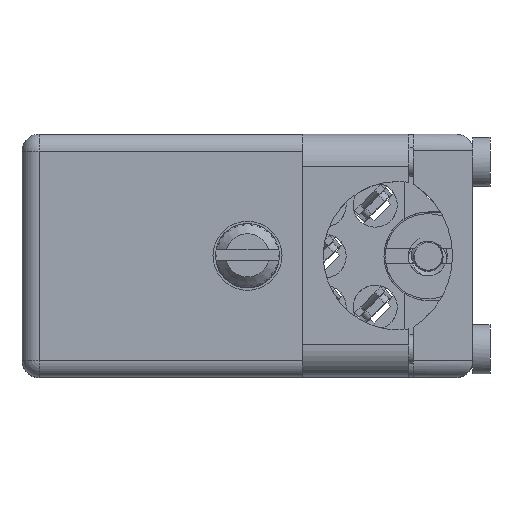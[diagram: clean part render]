
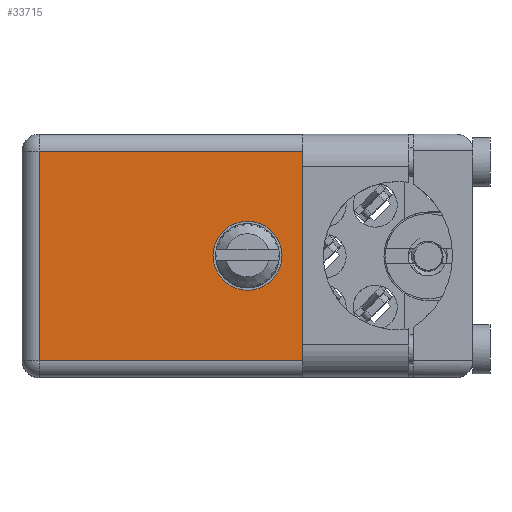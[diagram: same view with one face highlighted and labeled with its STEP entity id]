
A CAD part, top view. The second image highlights one B-rep face of the part: STEP entity #33715.
In plain terms, the highlighted face is planar.
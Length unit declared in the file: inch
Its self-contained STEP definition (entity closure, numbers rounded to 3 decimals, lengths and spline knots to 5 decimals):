
#2280 = VECTOR ( 'NONE', #78343, 39.37008 ) ;
#4469 = AXIS2_PLACEMENT_3D ( 'NONE', #117128, #179410, #145827 ) ;
#11707 = VECTOR ( 'NONE', #194479, 39.37008 ) ;
#15345 = ORIENTED_EDGE ( 'NONE', *, *, #191166, .F. ) ;
#16782 = ORIENTED_EDGE ( 'NONE', *, *, #192818, .F. ) ;
#17512 = AXIS2_PLACEMENT_3D ( 'NONE', #48209, #168682, #169655 ) ;
#18104 = CARTESIAN_POINT ( 'NONE',  ( 0., 0.906, -0.665 ) ) ;
#18209 = CARTESIAN_POINT ( 'NONE',  ( 0.05, 0.906, -0.715 ) ) ;
#19798 = CIRCLE ( 'NONE', #4469, 0.1015 ) ;
#19978 = VECTOR ( 'NONE', #87332, 39.37008 ) ;
#22488 = VERTEX_POINT ( 'NONE', #194819 ) ;
#24714 = LINE ( 'NONE', #98712, #146608 ) ;
#26294 = VERTEX_POINT ( 'NONE', #91456 ) ;
#27596 = LINE ( 'NONE', #102563, #11707 ) ;
#33715 = ADVANCED_FACE ( 'NONE', ( #63022, #94491 ), #183495, .T. ) ;
#39532 = DIRECTION ( 'NONE',  ( 0., 0., 1. ) ) ;
#39590 = CIRCLE ( 'NONE', #86900, 0.1015 ) ;
#40896 = VERTEX_POINT ( 'NONE', #136985 ) ;
#42227 = CARTESIAN_POINT ( 'NONE',  ( 0.05, 0.906, -0.05 ) ) ;
#43922 = LINE ( 'NONE', #132750, #19978 ) ;
#44995 = ORIENTED_EDGE ( 'NONE', *, *, #147206, .T. ) ;
#45551 = ORIENTED_EDGE ( 'NONE', *, *, #162852, .T. ) ;
#46807 = VECTOR ( 'NONE', #107483, 39.37008 ) ;
#46861 = LINE ( 'NONE', #169249, #115347 ) ;
#48209 = CARTESIAN_POINT ( 'NONE',  ( 0., 0.906, -0.715 ) ) ;
#51834 = DIRECTION ( 'NONE',  ( 1., 0., 0. ) ) ;
#62132 = LINE ( 'NONE', #122316, #46807 ) ;
#62166 = CARTESIAN_POINT ( 'NONE',  ( 1.15, 0.906, -0.6025 ) ) ;
#63022 = FACE_OUTER_BOUND ( 'NONE', #148347, .T. ) ;
#70532 = CARTESIAN_POINT ( 'NONE',  ( 1.15, 0.906, -0.05 ) ) ;
#73700 = VECTOR ( 'NONE', #51834, 39.37008 ) ;
#76303 = DIRECTION ( 'NONE',  ( 0., 0., 1. ) ) ;
#76359 = EDGE_CURVE ( 'NONE', #112661, #138164, #27596, .T. ) ;
#78343 = DIRECTION ( 'NONE',  ( -1., 0., 0. ) ) ;
#79406 = VERTEX_POINT ( 'NONE', #148824 ) ;
#80008 = VECTOR ( 'NONE', #141597, 39.37008 ) ;
#80374 = LINE ( 'NONE', #18209, #80008 ) ;
#84401 = CARTESIAN_POINT ( 'NONE',  ( 1.15, 0.906, -0.1125 ) ) ;
#84793 = ORIENTED_EDGE ( 'NONE', *, *, #152668, .F. ) ;
#85545 = VERTEX_POINT ( 'NONE', #157848 ) ;
#86900 = AXIS2_PLACEMENT_3D ( 'NONE', #109773, #125562, #76303 ) ;
#87332 = DIRECTION ( 'NONE',  ( 1., 0., 0. ) ) ;
#91456 = CARTESIAN_POINT ( 'NONE',  ( 0.865, 0.906, -0.6025 ) ) ;
#93102 = LINE ( 'NONE', #18104, #2280 ) ;
#93901 = ORIENTED_EDGE ( 'NONE', *, *, #76359, .T. ) ;
#94491 = FACE_BOUND ( 'NONE', #98132, .T. ) ;
#98132 = EDGE_LOOP ( 'NONE', ( #165272, #15345 ) ) ;
#98712 = CARTESIAN_POINT ( 'NONE',  ( 1.15, 0.906, -0.715 ) ) ;
#102563 = CARTESIAN_POINT ( 'NONE',  ( 0.865, 0.906, -0.1125 ) ) ;
#105263 = ORIENTED_EDGE ( 'NONE', *, *, #132419, .T. ) ;
#107483 = DIRECTION ( 'NONE',  ( 0., 0., -1. ) ) ;
#109773 = CARTESIAN_POINT ( 'NONE',  ( 0.6625, 0.906, -0.3575 ) ) ;
#112661 = VERTEX_POINT ( 'NONE', #84401 ) ;
#115347 = VECTOR ( 'NONE', #184052, 39.37008 ) ;
#117128 = CARTESIAN_POINT ( 'NONE',  ( 0.6625, 0.906, -0.3575 ) ) ;
#118645 = EDGE_CURVE ( 'NONE', #138164, #26294, #62132, .T. ) ;
#122316 = CARTESIAN_POINT ( 'NONE',  ( 0.865, 0.906, -0.1125 ) ) ;
#125562 = DIRECTION ( 'NONE',  ( 0., 1., 0. ) ) ;
#129329 = EDGE_CURVE ( 'NONE', #182599, #40896, #160449, .T. ) ;
#132419 = EDGE_CURVE ( 'NONE', #143278, #182599, #80374, .T. ) ;
#132750 = CARTESIAN_POINT ( 'NONE',  ( 0.865, 0.906, -0.6025 ) ) ;
#136495 = ORIENTED_EDGE ( 'NONE', *, *, #118645, .T. ) ;
#136985 = CARTESIAN_POINT ( 'NONE',  ( 1.15, 0.906, -0.05 ) ) ;
#138164 = VERTEX_POINT ( 'NONE', #168419 ) ;
#141597 = DIRECTION ( 'NONE',  ( 0., 0., 1. ) ) ;
#143278 = VERTEX_POINT ( 'NONE', #155475 ) ;
#145827 = DIRECTION ( 'NONE',  ( 0., 0., 1. ) ) ;
#146608 = VECTOR ( 'NONE', #39532, 39.37008 ) ;
#147206 = EDGE_CURVE ( 'NONE', #26294, #183003, #43922, .T. ) ;
#148347 = EDGE_LOOP ( 'NONE', ( #105263, #151082, #16782, #93901, #136495, #44995, #84793, #45551 ) ) ;
#148824 = CARTESIAN_POINT ( 'NONE',  ( 0.6625, 0.906, -0.459 ) ) ;
#151082 = ORIENTED_EDGE ( 'NONE', *, *, #129329, .T. ) ;
#152668 = EDGE_CURVE ( 'NONE', #22488, #183003, #24714, .T. ) ;
#155475 = CARTESIAN_POINT ( 'NONE',  ( 0.05, 0.906, -0.665 ) ) ;
#157848 = CARTESIAN_POINT ( 'NONE',  ( 0.6625, 0.906, -0.256 ) ) ;
#160449 = LINE ( 'NONE', #70532, #73700 ) ;
#162852 = EDGE_CURVE ( 'NONE', #22488, #143278, #93102, .T. ) ;
#165272 = ORIENTED_EDGE ( 'NONE', *, *, #177935, .F. ) ;
#168419 = CARTESIAN_POINT ( 'NONE',  ( 0.865, 0.906, -0.1125 ) ) ;
#168682 = DIRECTION ( 'NONE',  ( 0., 1., 0. ) ) ;
#169249 = CARTESIAN_POINT ( 'NONE',  ( 1.15, 0.906, -0.715 ) ) ;
#169655 = DIRECTION ( 'NONE',  ( 0., 0., 1. ) ) ;
#177935 = EDGE_CURVE ( 'NONE', #85545, #79406, #19798, .T. ) ;
#179410 = DIRECTION ( 'NONE',  ( 0., 1., 0. ) ) ;
#182599 = VERTEX_POINT ( 'NONE', #42227 ) ;
#183003 = VERTEX_POINT ( 'NONE', #62166 ) ;
#183495 = PLANE ( 'NONE',  #17512 ) ;
#184052 = DIRECTION ( 'NONE',  ( 0., 0., 1. ) ) ;
#191166 = EDGE_CURVE ( 'NONE', #79406, #85545, #39590, .T. ) ;
#192818 = EDGE_CURVE ( 'NONE', #112661, #40896, #46861, .T. ) ;
#194479 = DIRECTION ( 'NONE',  ( -1., 0., 0. ) ) ;
#194819 = CARTESIAN_POINT ( 'NONE',  ( 1.15, 0.906, -0.665 ) ) ;
